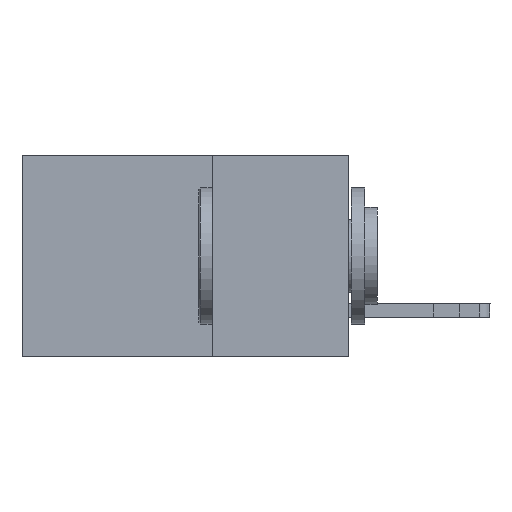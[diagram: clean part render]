
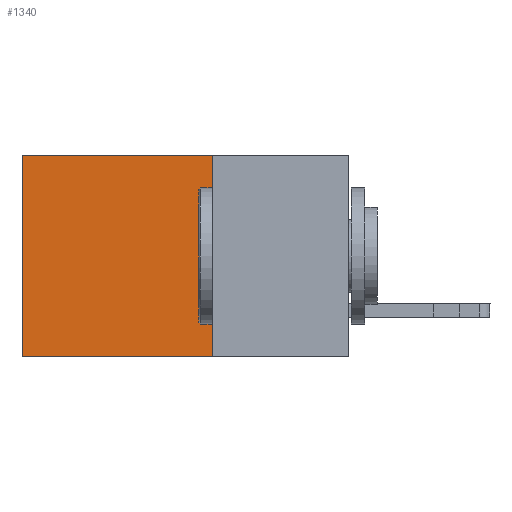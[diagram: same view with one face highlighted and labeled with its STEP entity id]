
A CAD part, left-side view. The second image highlights one B-rep face of the part: STEP entity #1340.
In plain terms, the highlighted planar face has unit normal (-1, 0, 0).
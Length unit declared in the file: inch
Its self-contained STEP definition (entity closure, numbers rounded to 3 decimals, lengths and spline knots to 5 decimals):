
#1030 = EDGE_CURVE ( 'NONE', #3297, #17855, #15092, .T. ) ;
#1340 = ADVANCED_FACE ( 'NONE', ( #13462 ), #10500, .F. ) ;
#2164 = DIRECTION ( 'NONE',  ( 0., 1., 0. ) ) ;
#3297 = VERTEX_POINT ( 'NONE', #13852 ) ;
#3624 = VERTEX_POINT ( 'NONE', #8448 ) ;
#3994 = CARTESIAN_POINT ( 'NONE',  ( 0.2615, 0.25, -0.37 ) ) ;
#5155 = ORIENTED_EDGE ( 'NONE', *, *, #1030, .F. ) ;
#5889 = DIRECTION ( 'NONE',  ( 0., 0., -1. ) ) ;
#6410 = CARTESIAN_POINT ( 'NONE',  ( 0.2615, 0.25, -0.37 ) ) ;
#7072 = EDGE_LOOP ( 'NONE', ( #17403, #5155, #19102, #11954 ) ) ;
#7850 = CARTESIAN_POINT ( 'NONE',  ( 0.2615, 0.6, -0.37 ) ) ;
#7947 = DIRECTION ( 'NONE',  ( 0., 0., -1. ) ) ;
#8448 = CARTESIAN_POINT ( 'NONE',  ( 0.2615, 0.6, 0. ) ) ;
#9401 = DIRECTION ( 'NONE',  ( 0., 1., 0. ) ) ;
#10500 = PLANE ( 'NONE',  #11559 ) ;
#11033 = CARTESIAN_POINT ( 'NONE',  ( 0.2615, 0.25, 0. ) ) ;
#11151 = VECTOR ( 'NONE', #2164, 39.37008 ) ;
#11559 = AXIS2_PLACEMENT_3D ( 'NONE', #3994, #18769, #5889 ) ;
#11706 = VECTOR ( 'NONE', #7947, 39.37008 ) ;
#11954 = ORIENTED_EDGE ( 'NONE', *, *, #19143, .T. ) ;
#12308 = LINE ( 'NONE', #16785, #15770 ) ;
#13071 = VECTOR ( 'NONE', #14804, 39.37008 ) ;
#13440 = EDGE_CURVE ( 'NONE', #3624, #17855, #16790, .T. ) ;
#13462 = FACE_OUTER_BOUND ( 'NONE', #7072, .T. ) ;
#13696 = EDGE_CURVE ( 'NONE', #17927, #3297, #16090, .T. ) ;
#13852 = CARTESIAN_POINT ( 'NONE',  ( 0.2615, 0.25, -0.37 ) ) ;
#14804 = DIRECTION ( 'NONE',  ( 0., 0., -1. ) ) ;
#15092 = LINE ( 'NONE', #18036, #11151 ) ;
#15770 = VECTOR ( 'NONE', #9401, 39.37008 ) ;
#16090 = LINE ( 'NONE', #6410, #11706 ) ;
#16785 = CARTESIAN_POINT ( 'NONE',  ( 0.2615, 0.25, 0. ) ) ;
#16790 = LINE ( 'NONE', #19234, #13071 ) ;
#17403 = ORIENTED_EDGE ( 'NONE', *, *, #13440, .T. ) ;
#17855 = VERTEX_POINT ( 'NONE', #7850 ) ;
#17927 = VERTEX_POINT ( 'NONE', #11033 ) ;
#18036 = CARTESIAN_POINT ( 'NONE',  ( 0.2615, 0.25, -0.37 ) ) ;
#18769 = DIRECTION ( 'NONE',  ( 1., 0., 0. ) ) ;
#19102 = ORIENTED_EDGE ( 'NONE', *, *, #13696, .F. ) ;
#19143 = EDGE_CURVE ( 'NONE', #17927, #3624, #12308, .T. ) ;
#19234 = CARTESIAN_POINT ( 'NONE',  ( 0.2615, 0.6, -0.37 ) ) ;
